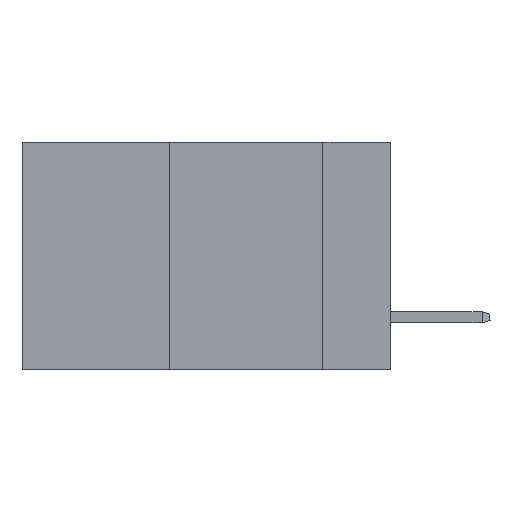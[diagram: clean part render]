
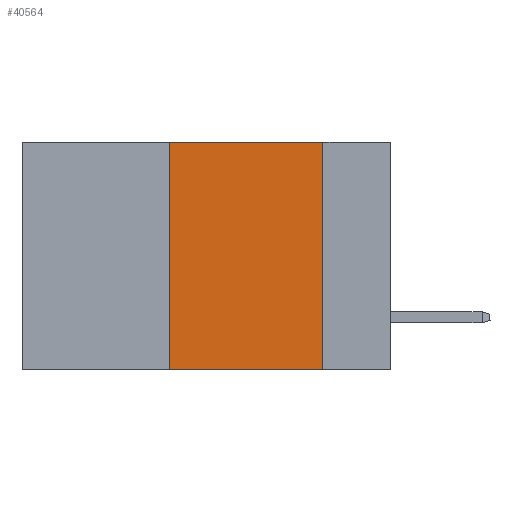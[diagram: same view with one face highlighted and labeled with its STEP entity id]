
A CAD part, left-side view. The second image highlights one B-rep face of the part: STEP entity #40564.
In plain terms, the highlighted planar face has unit normal (-1, 0, 0).
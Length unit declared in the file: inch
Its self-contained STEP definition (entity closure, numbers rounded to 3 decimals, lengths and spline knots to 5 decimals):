
#72 = ORIENTED_EDGE ( 'NONE', *, *, #14986, .F. ) ;
#583 = VECTOR ( 'NONE', #44732, 39.37008 ) ;
#1672 = FACE_OUTER_BOUND ( 'NONE', #9946, .T. ) ;
#1757 = EDGE_CURVE ( 'NONE', #22379, #6307, #10915, .T. ) ;
#2916 = CARTESIAN_POINT ( 'NONE',  ( 0., 0.11, 0. ) ) ;
#2925 = LINE ( 'NONE', #4031, #31142 ) ;
#3848 = EDGE_CURVE ( 'NONE', #12332, #4492, #2925, .T. ) ;
#4031 = CARTESIAN_POINT ( 'NONE',  ( 0., 0.36, 0. ) ) ;
#4492 = VERTEX_POINT ( 'NONE', #23383 ) ;
#6307 = VERTEX_POINT ( 'NONE', #7408 ) ;
#7408 = CARTESIAN_POINT ( 'NONE',  ( 0., 0.11, -0.37 ) ) ;
#8679 = DIRECTION ( 'NONE',  ( 0., -1., 0. ) ) ;
#9229 = AXIS2_PLACEMENT_3D ( 'NONE', #43300, #46959, #24669 ) ;
#9946 = EDGE_LOOP ( 'NONE', ( #17697, #72, #25923, #28617 ) ) ;
#10915 = LINE ( 'NONE', #2916, #583 ) ;
#11296 = CARTESIAN_POINT ( 'NONE',  ( 0., 0.36, -0.37 ) ) ;
#12332 = VERTEX_POINT ( 'NONE', #11296 ) ;
#14644 = LINE ( 'NONE', #19966, #33670 ) ;
#14699 = EDGE_CURVE ( 'NONE', #12332, #6307, #14644, .T. ) ;
#14986 = EDGE_CURVE ( 'NONE', #4492, #22379, #20595, .T. ) ;
#16978 = PLANE ( 'NONE',  #9229 ) ;
#17697 = ORIENTED_EDGE ( 'NONE', *, *, #1757, .F. ) ;
#19415 = VECTOR ( 'NONE', #44227, 39.37008 ) ;
#19966 = CARTESIAN_POINT ( 'NONE',  ( 0., 0.6, -0.37 ) ) ;
#20595 = LINE ( 'NONE', #25650, #19415 ) ;
#22379 = VERTEX_POINT ( 'NONE', #41686 ) ;
#23383 = CARTESIAN_POINT ( 'NONE',  ( 0., 0.36, 0. ) ) ;
#24669 = DIRECTION ( 'NONE',  ( 0., 0., -1. ) ) ;
#25650 = CARTESIAN_POINT ( 'NONE',  ( 0., 0.6, 0. ) ) ;
#25923 = ORIENTED_EDGE ( 'NONE', *, *, #3848, .F. ) ;
#28617 = ORIENTED_EDGE ( 'NONE', *, *, #14699, .T. ) ;
#30874 = DIRECTION ( 'NONE',  ( 0., 0., 1. ) ) ;
#31142 = VECTOR ( 'NONE', #30874, 39.37008 ) ;
#33670 = VECTOR ( 'NONE', #8679, 39.37008 ) ;
#40564 = ADVANCED_FACE ( 'NONE', ( #1672 ), #16978, .F. ) ;
#41686 = CARTESIAN_POINT ( 'NONE',  ( 0., 0.11, 0. ) ) ;
#43300 = CARTESIAN_POINT ( 'NONE',  ( 0., 0.6, 0. ) ) ;
#44227 = DIRECTION ( 'NONE',  ( 0., -1., 0. ) ) ;
#44732 = DIRECTION ( 'NONE',  ( 0., 0., -1. ) ) ;
#46959 = DIRECTION ( 'NONE',  ( 1., 0., 0. ) ) ;
